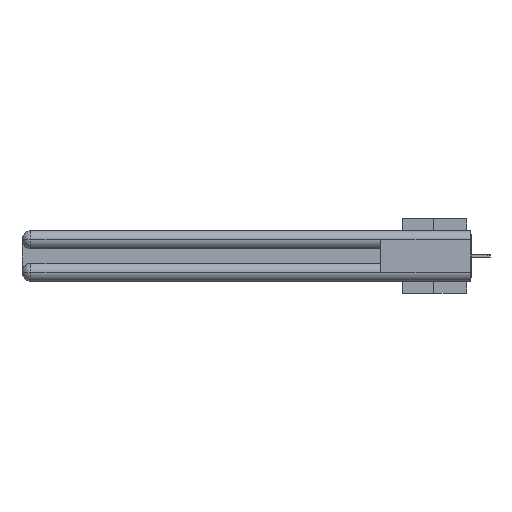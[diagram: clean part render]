
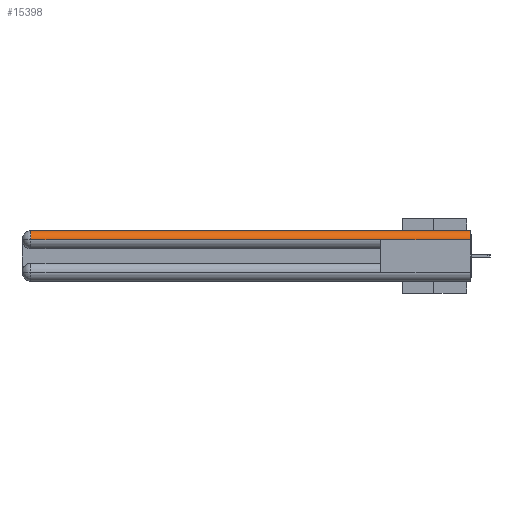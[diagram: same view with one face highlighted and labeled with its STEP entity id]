
A CAD part, left-side view. The second image highlights one B-rep face of the part: STEP entity #15398.
In plain terms, the highlighted cylindrical face has radius 1.562 mm (diameter 3.124 mm), a partial arc.
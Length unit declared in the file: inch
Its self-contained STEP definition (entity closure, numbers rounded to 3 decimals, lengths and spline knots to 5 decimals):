
#253 = DIRECTION ( 'NONE',  ( 0., 0., 1. ) ) ;
#675 = LINE ( 'NONE', #14082, #15345 ) ;
#787 = VECTOR ( 'NONE', #2847, 39.37008 ) ;
#812 = ORIENTED_EDGE ( 'NONE', *, *, #17268, .F. ) ;
#1055 = CARTESIAN_POINT ( 'NONE',  ( 0.0615, 0., -0.0615 ) ) ;
#2132 = LINE ( 'NONE', #32311, #32190 ) ;
#2445 = DIRECTION ( 'NONE',  ( 0., -1., 0. ) ) ;
#2847 = DIRECTION ( 'NONE',  ( 0., 1., 0. ) ) ;
#4084 = DIRECTION ( 'NONE',  ( 1., 0., 0. ) ) ;
#5361 = AXIS2_PLACEMENT_3D ( 'NONE', #1055, #21546, #4084 ) ;
#5369 = CARTESIAN_POINT ( 'NONE',  ( 0., 0.6, -0.0615 ) ) ;
#5968 = ORIENTED_EDGE ( 'NONE', *, *, #30240, .T. ) ;
#8751 = ORIENTED_EDGE ( 'NONE', *, *, #14476, .F. ) ;
#10114 = VERTEX_POINT ( 'NONE', #32586 ) ;
#11085 = VERTEX_POINT ( 'NONE', #5369 ) ;
#11407 = VERTEX_POINT ( 'NONE', #24194 ) ;
#11829 = CIRCLE ( 'NONE', #5361, 0.0615 ) ;
#12890 = DIRECTION ( 'NONE',  ( 0., 0., 1. ) ) ;
#13879 = ORIENTED_EDGE ( 'NONE', *, *, #18567, .T. ) ;
#14082 = CARTESIAN_POINT ( 'NONE',  ( 0.0615, 0., 0. ) ) ;
#14476 = EDGE_CURVE ( 'NONE', #10114, #28556, #675, .T. ) ;
#14952 = DIRECTION ( 'NONE',  ( 0., -1., 0. ) ) ;
#15345 = VECTOR ( 'NONE', #2445, 39.37008 ) ;
#15398 = ADVANCED_FACE ( 'NONE', ( #16894 ), #15975, .T. ) ;
#15975 = CYLINDRICAL_SURFACE ( 'NONE', #33744, 0.0615 ) ;
#16894 = FACE_OUTER_BOUND ( 'NONE', #22727, .T. ) ;
#17268 = EDGE_CURVE ( 'NONE', #28556, #24035, #11829, .T. ) ;
#17813 = DIRECTION ( 'NONE',  ( 0., -1., 0. ) ) ;
#18567 = EDGE_CURVE ( 'NONE', #10114, #11407, #22188, .T. ) ;
#18626 = DIRECTION ( 'NONE',  ( 0., 1., 0. ) ) ;
#19610 = ORIENTED_EDGE ( 'NONE', *, *, #29671, .F. ) ;
#21546 = DIRECTION ( 'NONE',  ( 0., -1., 0. ) ) ;
#21987 = AXIS2_PLACEMENT_3D ( 'NONE', #35139, #17813, #253 ) ;
#22188 = CIRCLE ( 'NONE', #21987, 0.0615 ) ;
#22727 = EDGE_LOOP ( 'NONE', ( #8751, #13879, #5968, #19610, #812 ) ) ;
#24035 = VERTEX_POINT ( 'NONE', #30830 ) ;
#24131 = LINE ( 'NONE', #37652, #787 ) ;
#24194 = CARTESIAN_POINT ( 'NONE',  ( 0., 2.94, -0.0615 ) ) ;
#28556 = VERTEX_POINT ( 'NONE', #37720 ) ;
#29671 = EDGE_CURVE ( 'NONE', #24035, #11085, #24131, .T. ) ;
#30240 = EDGE_CURVE ( 'NONE', #11407, #11085, #2132, .T. ) ;
#30296 = CARTESIAN_POINT ( 'NONE',  ( 0.0615, 0., -0.0615 ) ) ;
#30830 = CARTESIAN_POINT ( 'NONE',  ( 0., 0., -0.0615 ) ) ;
#32190 = VECTOR ( 'NONE', #14952, 39.37008 ) ;
#32311 = CARTESIAN_POINT ( 'NONE',  ( 0., 3., -0.0615 ) ) ;
#32586 = CARTESIAN_POINT ( 'NONE',  ( 0.0615, 2.94, 0. ) ) ;
#33744 = AXIS2_PLACEMENT_3D ( 'NONE', #30296, #18626, #12890 ) ;
#35139 = CARTESIAN_POINT ( 'NONE',  ( 0.0615, 2.94, -0.0615 ) ) ;
#37652 = CARTESIAN_POINT ( 'NONE',  ( 0., 3., -0.0615 ) ) ;
#37720 = CARTESIAN_POINT ( 'NONE',  ( 0.0615, 0., 0. ) ) ;
